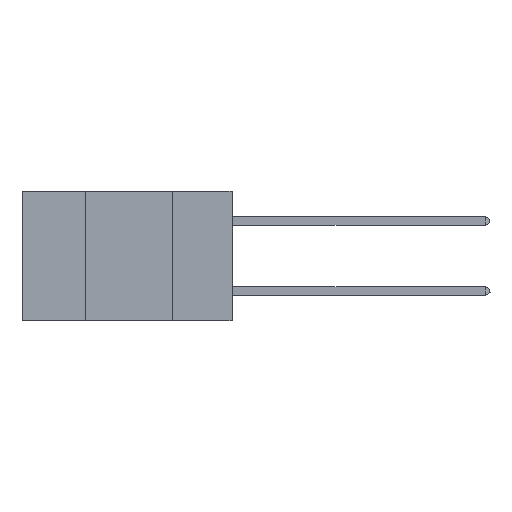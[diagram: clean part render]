
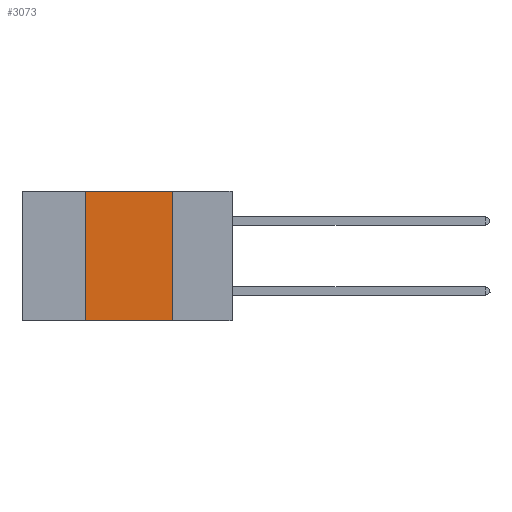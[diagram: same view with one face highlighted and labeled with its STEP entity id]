
A CAD part, left-side view. The second image highlights one B-rep face of the part: STEP entity #3073.
In plain terms, the highlighted planar face has unit normal (-1, 0, 0).
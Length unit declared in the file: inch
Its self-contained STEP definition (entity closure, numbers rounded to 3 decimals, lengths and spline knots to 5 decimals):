
#1496 = EDGE_CURVE ( 'NONE', #14315, #20577, #5160, .T. ) ;
#1540 = CARTESIAN_POINT ( 'NONE',  ( 0., 0.42, 0. ) ) ;
#1942 = ORIENTED_EDGE ( 'NONE', *, *, #23156, .T. ) ;
#2168 = CARTESIAN_POINT ( 'NONE',  ( 0., 0.6, 0. ) ) ;
#2464 = DIRECTION ( 'NONE',  ( 0., -1., 0. ) ) ;
#3073 = ADVANCED_FACE ( 'NONE', ( #15757 ), #14580, .F. ) ;
#4043 = VERTEX_POINT ( 'NONE', #31374 ) ;
#4277 = VECTOR ( 'NONE', #2464, 39.37008 ) ;
#4408 = DIRECTION ( 'NONE',  ( 0., 0., -1. ) ) ;
#5160 = LINE ( 'NONE', #29059, #9486 ) ;
#5919 = DIRECTION ( 'NONE',  ( 0., 0., -1. ) ) ;
#7044 = CARTESIAN_POINT ( 'NONE',  ( 0., 0.6, 0. ) ) ;
#8132 = CARTESIAN_POINT ( 'NONE',  ( 0., 0.42, -0.37 ) ) ;
#9486 = VECTOR ( 'NONE', #31184, 39.37008 ) ;
#10972 = LINE ( 'NONE', #17645, #4277 ) ;
#14205 = CARTESIAN_POINT ( 'NONE',  ( 0., 0.17, 0. ) ) ;
#14243 = LINE ( 'NONE', #2168, #25017 ) ;
#14315 = VERTEX_POINT ( 'NONE', #8132 ) ;
#14580 = PLANE ( 'NONE',  #15369 ) ;
#15286 = ORIENTED_EDGE ( 'NONE', *, *, #1496, .F. ) ;
#15299 = VECTOR ( 'NONE', #4408, 39.37008 ) ;
#15369 = AXIS2_PLACEMENT_3D ( 'NONE', #7044, #30816, #5919 ) ;
#15757 = FACE_OUTER_BOUND ( 'NONE', #26261, .T. ) ;
#17645 = CARTESIAN_POINT ( 'NONE',  ( 0., 0.6, -0.37 ) ) ;
#20577 = VERTEX_POINT ( 'NONE', #1540 ) ;
#22628 = DIRECTION ( 'NONE',  ( 0., -1., 0. ) ) ;
#22834 = VERTEX_POINT ( 'NONE', #14205 ) ;
#23156 = EDGE_CURVE ( 'NONE', #14315, #4043, #10972, .T. ) ;
#24220 = EDGE_CURVE ( 'NONE', #22834, #4043, #28846, .T. ) ;
#24833 = CARTESIAN_POINT ( 'NONE',  ( 0., 0.17, 0. ) ) ;
#25017 = VECTOR ( 'NONE', #22628, 39.37008 ) ;
#26261 = EDGE_LOOP ( 'NONE', ( #30351, #28221, #15286, #1942 ) ) ;
#28221 = ORIENTED_EDGE ( 'NONE', *, *, #28318, .F. ) ;
#28318 = EDGE_CURVE ( 'NONE', #20577, #22834, #14243, .T. ) ;
#28846 = LINE ( 'NONE', #24833, #15299 ) ;
#29059 = CARTESIAN_POINT ( 'NONE',  ( 0., 0.42, 0. ) ) ;
#30351 = ORIENTED_EDGE ( 'NONE', *, *, #24220, .F. ) ;
#30816 = DIRECTION ( 'NONE',  ( 1., 0., 0. ) ) ;
#31184 = DIRECTION ( 'NONE',  ( 0., 0., 1. ) ) ;
#31374 = CARTESIAN_POINT ( 'NONE',  ( 0., 0.17, -0.37 ) ) ;
